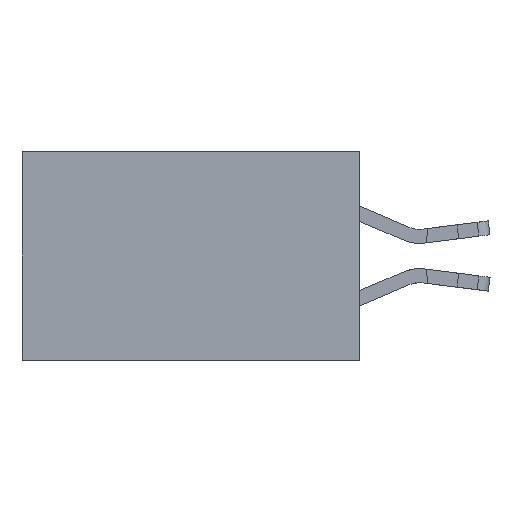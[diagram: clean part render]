
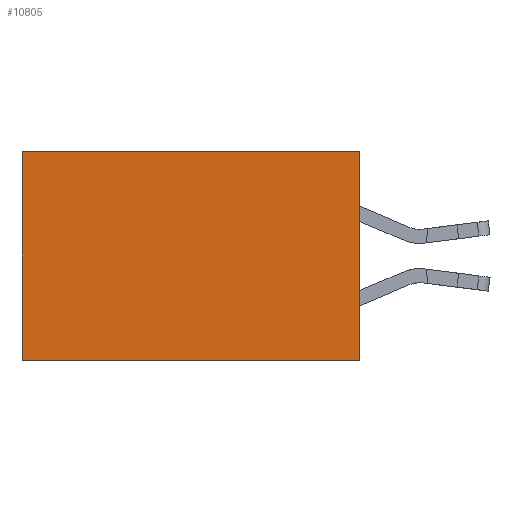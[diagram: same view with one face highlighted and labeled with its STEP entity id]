
A CAD part, left-side view. The second image highlights one B-rep face of the part: STEP entity #10805.
In plain terms, the highlighted planar face has unit normal (-1, 0, 0).
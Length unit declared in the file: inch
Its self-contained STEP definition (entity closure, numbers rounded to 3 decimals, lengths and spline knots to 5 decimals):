
#296 = VERTEX_POINT ( 'NONE', #6887 ) ;
#1008 = VERTEX_POINT ( 'NONE', #16492 ) ;
#1769 = FACE_OUTER_BOUND ( 'NONE', #6520, .T. ) ;
#1841 = CARTESIAN_POINT ( 'NONE',  ( 0.2875, 0.6, 0. ) ) ;
#2417 = AXIS2_PLACEMENT_3D ( 'NONE', #15384, #20480, #10305 ) ;
#3742 = CARTESIAN_POINT ( 'NONE',  ( 0.2875, 0., 0. ) ) ;
#3855 = LINE ( 'NONE', #3742, #16559 ) ;
#4246 = CARTESIAN_POINT ( 'NONE',  ( 0.2875, 0., 0. ) ) ;
#5657 = LINE ( 'NONE', #21131, #14758 ) ;
#5797 = CARTESIAN_POINT ( 'NONE',  ( 0.2875, 0.6, -0.37 ) ) ;
#6400 = ORIENTED_EDGE ( 'NONE', *, *, #22149, .T. ) ;
#6520 = EDGE_LOOP ( 'NONE', ( #6400, #10330, #7211, #20577 ) ) ;
#6887 = CARTESIAN_POINT ( 'NONE',  ( 0.2875, 0.6, 0. ) ) ;
#7211 = ORIENTED_EDGE ( 'NONE', *, *, #10971, .F. ) ;
#8577 = PLANE ( 'NONE',  #2417 ) ;
#9564 = EDGE_CURVE ( 'NONE', #1008, #15256, #21328, .T. ) ;
#9919 = CARTESIAN_POINT ( 'NONE',  ( 0.2875, 0., -0.37 ) ) ;
#10305 = DIRECTION ( 'NONE',  ( 0., 0., -1. ) ) ;
#10330 = ORIENTED_EDGE ( 'NONE', *, *, #9564, .F. ) ;
#10805 = ADVANCED_FACE ( 'NONE', ( #1769 ), #8577, .F. ) ;
#10971 = EDGE_CURVE ( 'NONE', #19432, #1008, #3855, .T. ) ;
#12306 = VECTOR ( 'NONE', #21785, 39.37008 ) ;
#14111 = DIRECTION ( 'NONE',  ( 0., 0., -1. ) ) ;
#14377 = LINE ( 'NONE', #1841, #22311 ) ;
#14758 = VECTOR ( 'NONE', #17747, 39.37008 ) ;
#15256 = VERTEX_POINT ( 'NONE', #5797 ) ;
#15384 = CARTESIAN_POINT ( 'NONE',  ( 0.2875, 0., 0. ) ) ;
#16492 = CARTESIAN_POINT ( 'NONE',  ( 0.2875, 0., -0.37 ) ) ;
#16559 = VECTOR ( 'NONE', #14111, 39.37008 ) ;
#17481 = DIRECTION ( 'NONE',  ( 0., 0., -1. ) ) ;
#17747 = DIRECTION ( 'NONE',  ( 0., 1., 0. ) ) ;
#19432 = VERTEX_POINT ( 'NONE', #4246 ) ;
#19915 = EDGE_CURVE ( 'NONE', #19432, #296, #5657, .T. ) ;
#20480 = DIRECTION ( 'NONE',  ( 1., 0., 0. ) ) ;
#20577 = ORIENTED_EDGE ( 'NONE', *, *, #19915, .T. ) ;
#21131 = CARTESIAN_POINT ( 'NONE',  ( 0.2875, 0., 0. ) ) ;
#21328 = LINE ( 'NONE', #9919, #12306 ) ;
#21785 = DIRECTION ( 'NONE',  ( 0., 1., 0. ) ) ;
#22149 = EDGE_CURVE ( 'NONE', #296, #15256, #14377, .T. ) ;
#22311 = VECTOR ( 'NONE', #17481, 39.37008 ) ;
